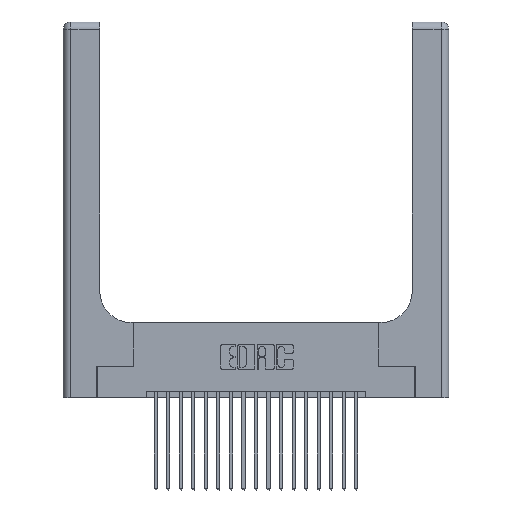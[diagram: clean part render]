
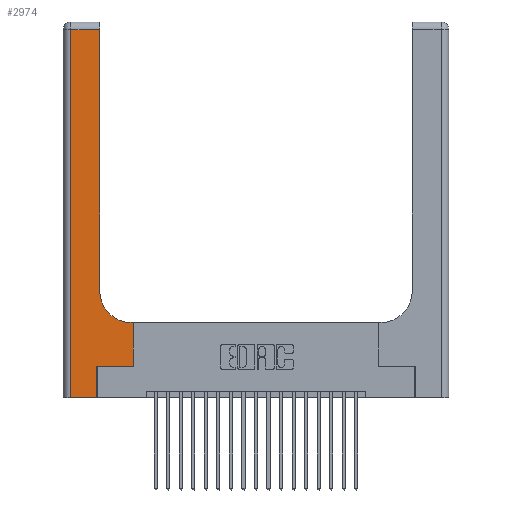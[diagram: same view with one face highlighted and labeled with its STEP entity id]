
A CAD part, top view. The second image highlights one B-rep face of the part: STEP entity #2974.
In plain terms, the highlighted planar face has unit normal (0, 0, 1).
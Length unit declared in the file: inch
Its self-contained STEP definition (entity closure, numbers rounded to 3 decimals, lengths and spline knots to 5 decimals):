
#304 = LINE ( 'NONE', #19262, #18069 ) ;
#478 = EDGE_CURVE ( 'NONE', #9612, #16986, #2757, .T. ) ;
#1294 = DIRECTION ( 'NONE',  ( -1., 0., 0. ) ) ;
#1395 = DIRECTION ( 'NONE',  ( 0., 0., -1. ) ) ;
#1458 = PLANE ( 'NONE',  #12049 ) ;
#2062 = DIRECTION ( 'NONE',  ( 0., 1., 0. ) ) ;
#2112 = CARTESIAN_POINT ( 'NONE',  ( 0., 3., 0.37 ) ) ;
#2428 = EDGE_CURVE ( 'NONE', #21271, #18303, #7684, .T. ) ;
#2757 = LINE ( 'NONE', #8400, #20723 ) ;
#2859 = FACE_OUTER_BOUND ( 'NONE', #5168, .T. ) ;
#2974 = ADVANCED_FACE ( 'NONE', ( #2859 ), #1458, .F. ) ;
#2989 = VECTOR ( 'NONE', #11223, 39.37008 ) ;
#3213 = VERTEX_POINT ( 'NONE', #16311 ) ;
#3816 = ORIENTED_EDGE ( 'NONE', *, *, #20496, .T. ) ;
#3839 = EDGE_CURVE ( 'NONE', #17503, #17119, #10767, .T. ) ;
#4070 = AXIS2_PLACEMENT_3D ( 'NONE', #15085, #4755, #16730 ) ;
#4121 = DIRECTION ( 'NONE',  ( 1., 0., 0. ) ) ;
#4646 = CARTESIAN_POINT ( 'NONE',  ( 0.5585, 0.25, 0.37 ) ) ;
#4755 = DIRECTION ( 'NONE',  ( 0., 0., -1. ) ) ;
#4939 = ORIENTED_EDGE ( 'NONE', *, *, #15512, .T. ) ;
#4977 = CARTESIAN_POINT ( 'NONE',  ( 0.269, 0., 0.37 ) ) ;
#5168 = EDGE_LOOP ( 'NONE', ( #3816, #4939, #19411, #20403, #19665, #7411, #19242, #6938, #20010 ) ) ;
#5445 = VERTEX_POINT ( 'NONE', #12010 ) ;
#5581 = CIRCLE ( 'NONE', #4070, 0.25 ) ;
#6938 = ORIENTED_EDGE ( 'NONE', *, *, #2428, .T. ) ;
#7257 = DIRECTION ( 'NONE',  ( -1., 0., 0. ) ) ;
#7411 = ORIENTED_EDGE ( 'NONE', *, *, #478, .T. ) ;
#7579 = DIRECTION ( 'NONE',  ( 0., -1., 0. ) ) ;
#7684 = LINE ( 'NONE', #11292, #2989 ) ;
#8400 = CARTESIAN_POINT ( 'NONE',  ( 0.269, 0.25, 0.37 ) ) ;
#8427 = DIRECTION ( 'NONE',  ( 1., 0., 0. ) ) ;
#9612 = VERTEX_POINT ( 'NONE', #15946 ) ;
#9733 = LINE ( 'NONE', #4646, #21816 ) ;
#10183 = CARTESIAN_POINT ( 'NONE',  ( 0.5415, 0.6, 0.37 ) ) ;
#10496 = LINE ( 'NONE', #10821, #14499 ) ;
#10767 = LINE ( 'NONE', #14462, #15317 ) ;
#10821 = CARTESIAN_POINT ( 'NONE',  ( 0.2915, 3., 0.37 ) ) ;
#11223 = DIRECTION ( 'NONE',  ( -1., 0., 0. ) ) ;
#11292 = CARTESIAN_POINT ( 'NONE',  ( 0.2915, 0.6, 0.37 ) ) ;
#11715 = EDGE_CURVE ( 'NONE', #16986, #21271, #9733, .T. ) ;
#12010 = CARTESIAN_POINT ( 'NONE',  ( 0.06, 2.94, 0.37 ) ) ;
#12049 = AXIS2_PLACEMENT_3D ( 'NONE', #2112, #1395, #1294 ) ;
#12683 = EDGE_CURVE ( 'NONE', #5445, #17503, #304, .T. ) ;
#13055 = CARTESIAN_POINT ( 'NONE',  ( 0.2915, 2.94, 0.37 ) ) ;
#13197 = VECTOR ( 'NONE', #21512, 39.37008 ) ;
#14420 = LINE ( 'NONE', #15788, #16960 ) ;
#14462 = CARTESIAN_POINT ( 'NONE',  ( 0., 0., 0.37 ) ) ;
#14499 = VECTOR ( 'NONE', #2062, 39.37008 ) ;
#14535 = EDGE_CURVE ( 'NONE', #18303, #3213, #5581, .T. ) ;
#14675 = CARTESIAN_POINT ( 'NONE',  ( 0.5585, 0.6, 0.37 ) ) ;
#15085 = CARTESIAN_POINT ( 'NONE',  ( 0.5415, 0.85, 0.37 ) ) ;
#15136 = VERTEX_POINT ( 'NONE', #13055 ) ;
#15317 = VECTOR ( 'NONE', #4121, 39.37008 ) ;
#15512 = EDGE_CURVE ( 'NONE', #15136, #5445, #14420, .T. ) ;
#15788 = CARTESIAN_POINT ( 'NONE',  ( 0., 2.94, 0.37 ) ) ;
#15946 = CARTESIAN_POINT ( 'NONE',  ( 0.269, 0.25, 0.37 ) ) ;
#16311 = CARTESIAN_POINT ( 'NONE',  ( 0.2915, 0.85, 0.37 ) ) ;
#16442 = CARTESIAN_POINT ( 'NONE',  ( 0.06, 0., 0.37 ) ) ;
#16730 = DIRECTION ( 'NONE',  ( 1., 0., 0. ) ) ;
#16960 = VECTOR ( 'NONE', #7257, 39.37008 ) ;
#16986 = VERTEX_POINT ( 'NONE', #21182 ) ;
#17119 = VERTEX_POINT ( 'NONE', #4977 ) ;
#17503 = VERTEX_POINT ( 'NONE', #16442 ) ;
#18069 = VECTOR ( 'NONE', #7579, 39.37008 ) ;
#18142 = CARTESIAN_POINT ( 'NONE',  ( 0.269, 0., 0.37 ) ) ;
#18303 = VERTEX_POINT ( 'NONE', #10183 ) ;
#19242 = ORIENTED_EDGE ( 'NONE', *, *, #11715, .T. ) ;
#19262 = CARTESIAN_POINT ( 'NONE',  ( 0.06, 3., 0.37 ) ) ;
#19411 = ORIENTED_EDGE ( 'NONE', *, *, #12683, .T. ) ;
#19665 = ORIENTED_EDGE ( 'NONE', *, *, #19873, .T. ) ;
#19873 = EDGE_CURVE ( 'NONE', #17119, #9612, #21797, .T. ) ;
#20010 = ORIENTED_EDGE ( 'NONE', *, *, #14535, .T. ) ;
#20403 = ORIENTED_EDGE ( 'NONE', *, *, #3839, .T. ) ;
#20496 = EDGE_CURVE ( 'NONE', #3213, #15136, #10496, .T. ) ;
#20723 = VECTOR ( 'NONE', #8427, 39.37008 ) ;
#21182 = CARTESIAN_POINT ( 'NONE',  ( 0.5585, 0.25, 0.37 ) ) ;
#21271 = VERTEX_POINT ( 'NONE', #14675 ) ;
#21447 = DIRECTION ( 'NONE',  ( 0., 1., 0. ) ) ;
#21512 = DIRECTION ( 'NONE',  ( 0., 1., 0. ) ) ;
#21797 = LINE ( 'NONE', #18142, #13197 ) ;
#21816 = VECTOR ( 'NONE', #21447, 39.37008 ) ;
